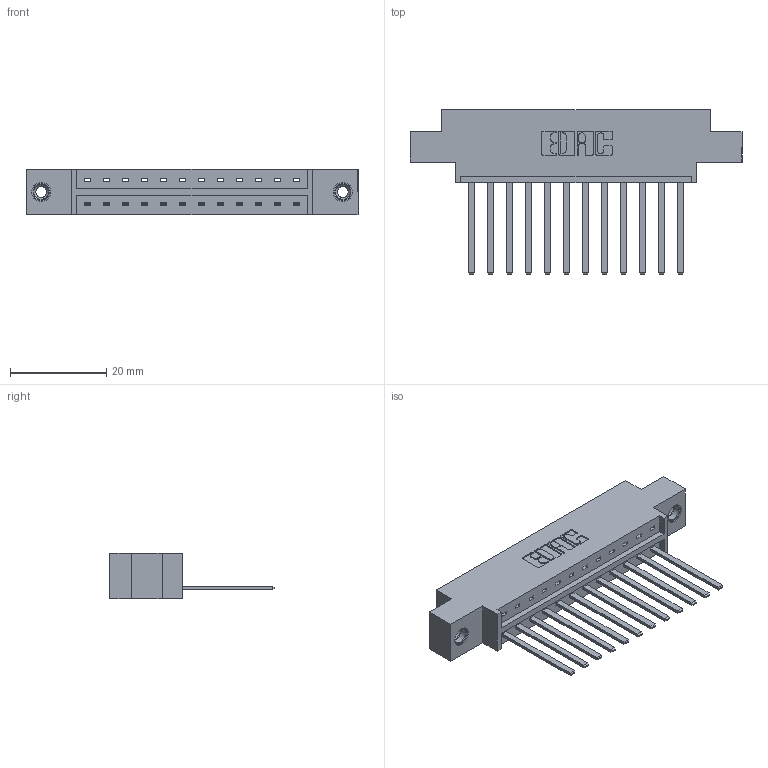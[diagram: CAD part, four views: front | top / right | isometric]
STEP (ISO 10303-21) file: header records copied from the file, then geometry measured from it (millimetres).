
FILE_DESCRIPTION (( 'STEP AP203' ), '1' );
FILE_NAME ('833-012-544-608.STEP', '2020-05-30T22:27:40', ( '' ), ( '' ), 'SwSTEP 2.0', 'SolidWorks 2020', '' );
FILE_SCHEMA (( 'CONFIG_CONTROL_DESIGN' ));
Length unit declared in the file: inch
Products named in the file (4): 345-250-001_345-250-003-102; 833-012-544-608; 833 Part_Offset - .156 Dia - TI; 345-292-001_345-293-144
Assembly tree (15 placements, depth 2):
  833-012-544-608
    833 Part_Offset - .156 Dia - TI
    345-292-001_345-293-144  x12
    345-250-001_345-250-003-102  x2
Bounding box: 69.09 x 34.3 x 9.4 mm (x, y, z)
Volume: 6598.9 mm3; surface area: 7619.2 mm2
Topology: 15 solids, 15 shells, 802 faces, 2355 edges, 1546 vertices
Faces by surface type: plane 562, cylinder 224, cone 12, torus 4
Entity records: 12350 total; most frequent: CARTESIAN_POINT 2117, ORIENTED_EDGE 2058, DIRECTION 1875, EDGE_CURVE 1029, VECTOR 885, LINE 885, VERTEX_POINT 680, AXIS2_PLACEMENT_3D 495
